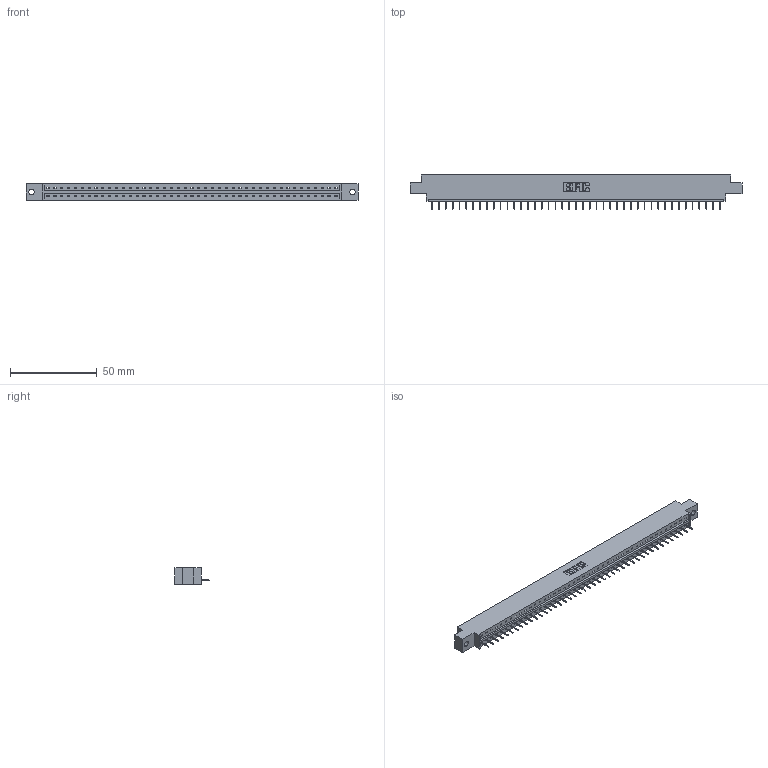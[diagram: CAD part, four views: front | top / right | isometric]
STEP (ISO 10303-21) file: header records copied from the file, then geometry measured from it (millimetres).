
FILE_DESCRIPTION (( 'STEP AP203' ), '1' );
FILE_NAME ('833-043-524-602.STEP', '2020-06-03T23:40:54', ( '' ), ( '' ), 'SwSTEP 2.0', 'SolidWorks 2020', '' );
FILE_SCHEMA (( 'CONFIG_CONTROL_DESIGN' ));
Length unit declared in the file: inch
Products named in the file (3): 833-043-524-602; 833 Part_Offset - .128 Dia; 345-292-001_345-293-124
Assembly tree (44 placements, depth 2):
  833-043-524-602
    833 Part_Offset - .128 Dia
    345-292-001_345-293-124  x43
Bounding box: 191.92 x 19.69 x 9.4 mm (x, y, z)
Volume: 18887.1 mm3; surface area: 19784 mm2
Topology: 44 solids, 44 shells, 2784 faces, 8063 edges, 5202 vertices
Faces by surface type: plane 2138, cylinder 646
Entity records: 26367 total; most frequent: CARTESIAN_POINT 4555, ORIENTED_EDGE 4534, DIRECTION 3841, EDGE_CURVE 2267, LINE 2143, VECTOR 2143, VERTEX_POINT 1506, AXIS2_PLACEMENT_3D 849
